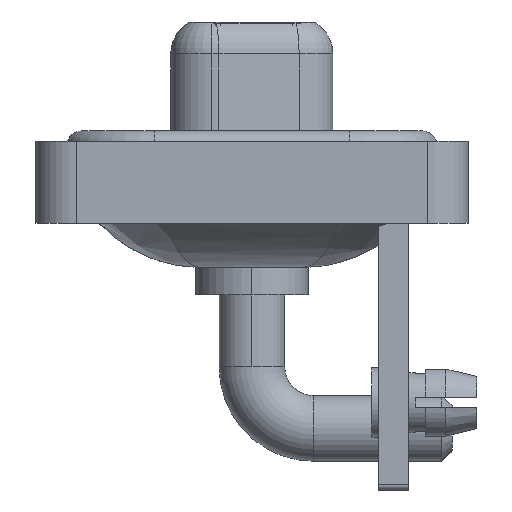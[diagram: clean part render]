
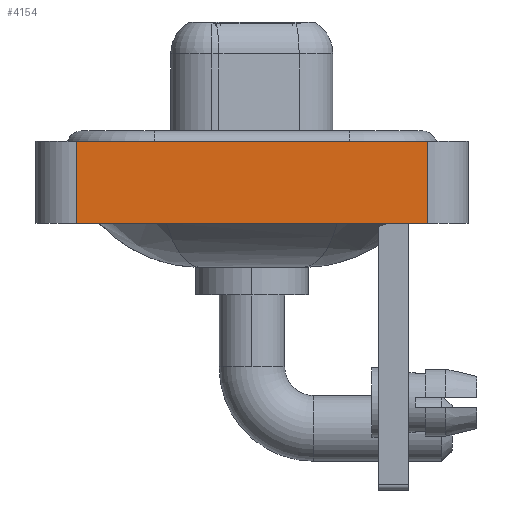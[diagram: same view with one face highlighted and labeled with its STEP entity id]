
A CAD part, left-side view. The second image highlights one B-rep face of the part: STEP entity #4154.
In plain terms, the highlighted planar face has unit normal (-1, 0, 0).
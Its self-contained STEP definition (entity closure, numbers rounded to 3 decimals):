
#350 = EDGE_CURVE ( 'NONE', #951, #14096, #14236, .T. ) ;
#951 = VERTEX_POINT ( 'NONE', #18037 ) ;
#1094 = VERTEX_POINT ( 'NONE', #12740 ) ;
#1258 = CARTESIAN_POINT ( 'NONE',  ( -7.25, 8.55, 0.4 ) ) ;
#2039 = EDGE_CURVE ( 'NONE', #14096, #1094, #9313, .T. ) ;
#2642 = DIRECTION ( 'NONE',  ( 0., 0., 1. ) ) ;
#4053 = EDGE_LOOP ( 'NONE', ( #10461, #5850, #12206, #11745 ) ) ;
#4154 = ADVANCED_FACE ( 'NONE', ( #4451 ), #12191, .T. ) ;
#4450 = DIRECTION ( 'NONE',  ( 0., -1., 0. ) ) ;
#4451 = FACE_OUTER_BOUND ( 'NONE', #4053, .T. ) ;
#4684 = LINE ( 'NONE', #10031, #9486 ) ;
#5850 = ORIENTED_EDGE ( 'NONE', *, *, #11887, .F. ) ;
#5998 = VERTEX_POINT ( 'NONE', #1258 ) ;
#6503 = VECTOR ( 'NONE', #2642, 1000. ) ;
#6833 = CARTESIAN_POINT ( 'NONE',  ( -7.25, 8.55, -3.6 ) ) ;
#7221 = CARTESIAN_POINT ( 'NONE',  ( -7.25, -8.55, -3.6 ) ) ;
#7359 = DIRECTION ( 'NONE',  ( 0., -1., 0. ) ) ;
#9074 = EDGE_CURVE ( 'NONE', #951, #5998, #13826, .T. ) ;
#9313 = LINE ( 'NONE', #9566, #6503 ) ;
#9486 = VECTOR ( 'NONE', #7359, 1000. ) ;
#9566 = CARTESIAN_POINT ( 'NONE',  ( -7.25, -8.55, -3.6 ) ) ;
#10031 = CARTESIAN_POINT ( 'NONE',  ( -7.25, -8.55, 0.4 ) ) ;
#10209 = AXIS2_PLACEMENT_3D ( 'NONE', #10807, #10450, #13300 ) ;
#10450 = DIRECTION ( 'NONE',  ( -1., 0., 0. ) ) ;
#10461 = ORIENTED_EDGE ( 'NONE', *, *, #2039, .T. ) ;
#10807 = CARTESIAN_POINT ( 'NONE',  ( -7.25, -8.55, -3.6 ) ) ;
#11460 = VECTOR ( 'NONE', #4450, 1000. ) ;
#11745 = ORIENTED_EDGE ( 'NONE', *, *, #350, .T. ) ;
#11887 = EDGE_CURVE ( 'NONE', #5998, #1094, #4684, .T. ) ;
#12191 = PLANE ( 'NONE',  #10209 ) ;
#12206 = ORIENTED_EDGE ( 'NONE', *, *, #9074, .F. ) ;
#12441 = DIRECTION ( 'NONE',  ( 0., 0., 1. ) ) ;
#12740 = CARTESIAN_POINT ( 'NONE',  ( -7.25, -8.55, 0.4 ) ) ;
#13288 = CARTESIAN_POINT ( 'NONE',  ( -7.25, -8.55, -3.6 ) ) ;
#13300 = DIRECTION ( 'NONE',  ( 0., 0., 1. ) ) ;
#13826 = LINE ( 'NONE', #6833, #14871 ) ;
#14096 = VERTEX_POINT ( 'NONE', #13288 ) ;
#14236 = LINE ( 'NONE', #7221, #11460 ) ;
#14871 = VECTOR ( 'NONE', #12441, 1000. ) ;
#18037 = CARTESIAN_POINT ( 'NONE',  ( -7.25, 8.55, -3.6 ) ) ;
